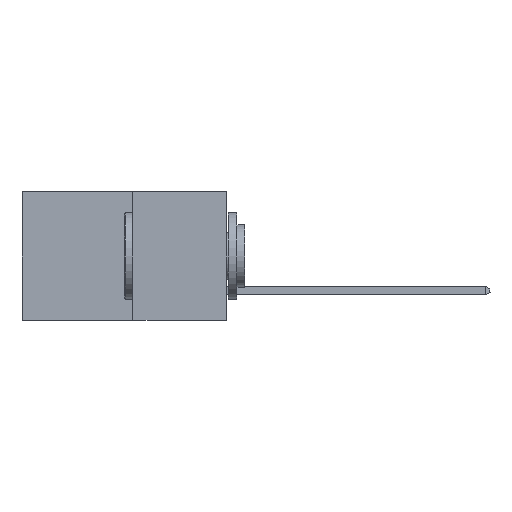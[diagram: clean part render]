
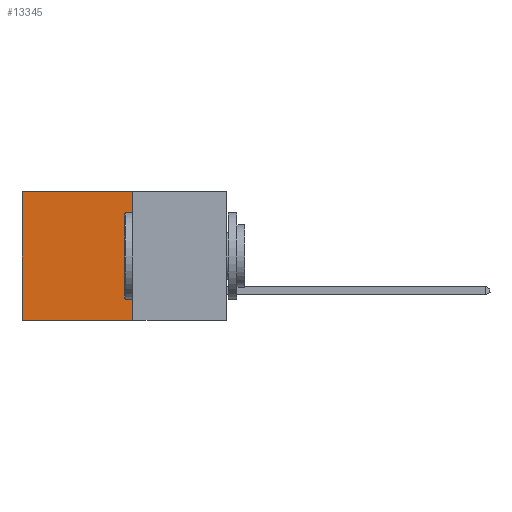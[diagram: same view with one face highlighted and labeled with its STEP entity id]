
A CAD part, left-side view. The second image highlights one B-rep face of the part: STEP entity #13345.
In plain terms, the highlighted planar face has unit normal (-1, 0, 0).
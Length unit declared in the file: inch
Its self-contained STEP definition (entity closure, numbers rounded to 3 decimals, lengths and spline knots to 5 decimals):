
#60 = DIRECTION ( 'NONE',  ( 0., 0., -1. ) ) ;
#470 = ORIENTED_EDGE ( 'NONE', *, *, #4799, .T. ) ;
#732 = CARTESIAN_POINT ( 'NONE',  ( 0.277, 0.59, -0.37 ) ) ;
#1503 = ORIENTED_EDGE ( 'NONE', *, *, #9412, .F. ) ;
#1650 = VECTOR ( 'NONE', #10841, 39.37008 ) ;
#2255 = ORIENTED_EDGE ( 'NONE', *, *, #2444, .T. ) ;
#2444 = EDGE_CURVE ( 'NONE', #15657, #10652, #9570, .T. ) ;
#3394 = DIRECTION ( 'NONE',  ( 0., 0., -1. ) ) ;
#3791 = ORIENTED_EDGE ( 'NONE', *, *, #13590, .F. ) ;
#3906 = VECTOR ( 'NONE', #3394, 39.37008 ) ;
#4441 = FACE_OUTER_BOUND ( 'NONE', #10620, .T. ) ;
#4799 = EDGE_CURVE ( 'NONE', #10652, #17440, #7360, .T. ) ;
#7198 = VECTOR ( 'NONE', #9578, 39.37008 ) ;
#7360 = LINE ( 'NONE', #732, #3906 ) ;
#9035 = DIRECTION ( 'NONE',  ( 1., 0., 0. ) ) ;
#9290 = LINE ( 'NONE', #9753, #16560 ) ;
#9412 = EDGE_CURVE ( 'NONE', #15833, #17440, #9290, .T. ) ;
#9570 = LINE ( 'NONE', #11003, #1650 ) ;
#9578 = DIRECTION ( 'NONE',  ( 0., 0., -1. ) ) ;
#9753 = CARTESIAN_POINT ( 'NONE',  ( 0.277, 0.27, -0.37 ) ) ;
#9847 = CARTESIAN_POINT ( 'NONE',  ( 0.277, 0.59, 0. ) ) ;
#10061 = CARTESIAN_POINT ( 'NONE',  ( 0.277, 0.59, -0.37 ) ) ;
#10620 = EDGE_LOOP ( 'NONE', ( #470, #1503, #3791, #2255 ) ) ;
#10652 = VERTEX_POINT ( 'NONE', #9847 ) ;
#10841 = DIRECTION ( 'NONE',  ( 0., 1., 0. ) ) ;
#11003 = CARTESIAN_POINT ( 'NONE',  ( 0.277, 0.27, 0. ) ) ;
#11098 = CARTESIAN_POINT ( 'NONE',  ( 0.277, 0.27, -0.37 ) ) ;
#11233 = LINE ( 'NONE', #11098, #7198 ) ;
#11275 = DIRECTION ( 'NONE',  ( 0., 1., 0. ) ) ;
#12773 = CARTESIAN_POINT ( 'NONE',  ( 0.277, 0.27, 0. ) ) ;
#13345 = ADVANCED_FACE ( 'NONE', ( #4441 ), #19006, .F. ) ;
#13590 = EDGE_CURVE ( 'NONE', #15657, #15833, #11233, .T. ) ;
#14685 = CARTESIAN_POINT ( 'NONE',  ( 0.277, 0.27, -0.37 ) ) ;
#15657 = VERTEX_POINT ( 'NONE', #12773 ) ;
#15833 = VERTEX_POINT ( 'NONE', #14685 ) ;
#16560 = VECTOR ( 'NONE', #11275, 39.37008 ) ;
#17440 = VERTEX_POINT ( 'NONE', #10061 ) ;
#17558 = AXIS2_PLACEMENT_3D ( 'NONE', #17702, #9035, #60 ) ;
#17702 = CARTESIAN_POINT ( 'NONE',  ( 0.277, 0.27, -0.37 ) ) ;
#19006 = PLANE ( 'NONE',  #17558 ) ;
